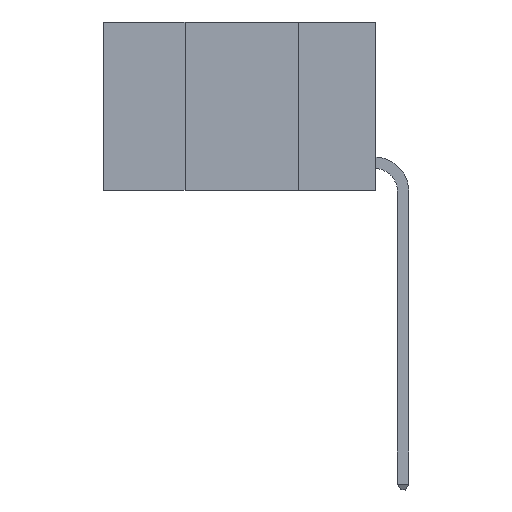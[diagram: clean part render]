
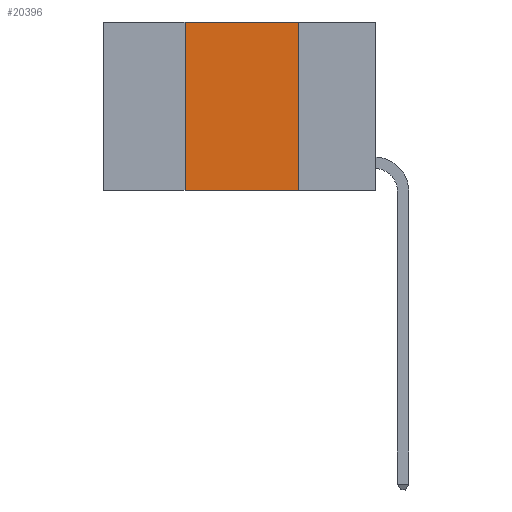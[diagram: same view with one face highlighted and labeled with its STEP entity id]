
A CAD part, left-side view. The second image highlights one B-rep face of the part: STEP entity #20396.
In plain terms, the highlighted planar face has unit normal (-1, 0, 0).
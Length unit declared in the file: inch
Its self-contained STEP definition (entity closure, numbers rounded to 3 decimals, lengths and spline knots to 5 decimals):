
#529 = CARTESIAN_POINT ( 'NONE',  ( 0., 0.42, -0.37 ) ) ;
#1071 = CARTESIAN_POINT ( 'NONE',  ( 0., 0.17, 0. ) ) ;
#1522 = CARTESIAN_POINT ( 'NONE',  ( 0., 0.6, -0.37 ) ) ;
#1681 = AXIS2_PLACEMENT_3D ( 'NONE', #2445, #4107, #15673 ) ;
#2064 = DIRECTION ( 'NONE',  ( 0., -1., 0. ) ) ;
#2176 = VECTOR ( 'NONE', #9682, 39.37008 ) ;
#2445 = CARTESIAN_POINT ( 'NONE',  ( 0., 0.6, 0. ) ) ;
#2550 = CARTESIAN_POINT ( 'NONE',  ( 0., 0.42, 0. ) ) ;
#2801 = EDGE_LOOP ( 'NONE', ( #10383, #14302, #15811, #20292 ) ) ;
#2963 = FACE_OUTER_BOUND ( 'NONE', #2801, .T. ) ;
#3199 = DIRECTION ( 'NONE',  ( 0., -1., 0. ) ) ;
#3222 = LINE ( 'NONE', #17884, #2176 ) ;
#3864 = VERTEX_POINT ( 'NONE', #15767 ) ;
#4107 = DIRECTION ( 'NONE',  ( 1., 0., 0. ) ) ;
#4428 = VECTOR ( 'NONE', #2064, 39.37008 ) ;
#5210 = VERTEX_POINT ( 'NONE', #1071 ) ;
#7799 = VECTOR ( 'NONE', #3199, 39.37008 ) ;
#8317 = LINE ( 'NONE', #1522, #7799 ) ;
#9337 = LINE ( 'NONE', #2550, #18604 ) ;
#9682 = DIRECTION ( 'NONE',  ( 0., 0., -1. ) ) ;
#10383 = ORIENTED_EDGE ( 'NONE', *, *, #21279, .F. ) ;
#12361 = PLANE ( 'NONE',  #1681 ) ;
#12853 = EDGE_CURVE ( 'NONE', #16641, #16740, #8317, .T. ) ;
#14124 = DIRECTION ( 'NONE',  ( 0., 0., 1. ) ) ;
#14302 = ORIENTED_EDGE ( 'NONE', *, *, #17178, .F. ) ;
#15673 = DIRECTION ( 'NONE',  ( 0., 0., -1. ) ) ;
#15767 = CARTESIAN_POINT ( 'NONE',  ( 0., 0.42, 0. ) ) ;
#15811 = ORIENTED_EDGE ( 'NONE', *, *, #18019, .F. ) ;
#16641 = VERTEX_POINT ( 'NONE', #529 ) ;
#16740 = VERTEX_POINT ( 'NONE', #19223 ) ;
#16879 = CARTESIAN_POINT ( 'NONE',  ( 0., 0.6, 0. ) ) ;
#17178 = EDGE_CURVE ( 'NONE', #3864, #5210, #17609, .T. ) ;
#17609 = LINE ( 'NONE', #16879, #4428 ) ;
#17884 = CARTESIAN_POINT ( 'NONE',  ( 0., 0.17, 0. ) ) ;
#18019 = EDGE_CURVE ( 'NONE', #16641, #3864, #9337, .T. ) ;
#18604 = VECTOR ( 'NONE', #14124, 39.37008 ) ;
#19223 = CARTESIAN_POINT ( 'NONE',  ( 0., 0.17, -0.37 ) ) ;
#20292 = ORIENTED_EDGE ( 'NONE', *, *, #12853, .T. ) ;
#20396 = ADVANCED_FACE ( 'NONE', ( #2963 ), #12361, .F. ) ;
#21279 = EDGE_CURVE ( 'NONE', #5210, #16740, #3222, .T. ) ;
